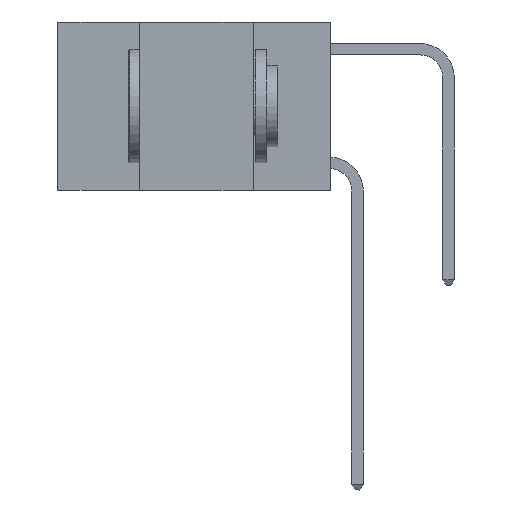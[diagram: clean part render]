
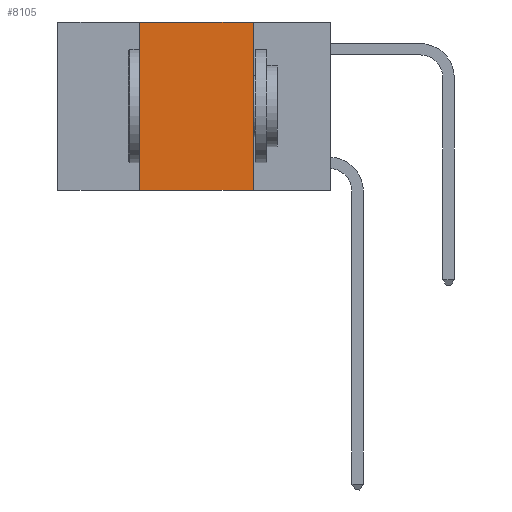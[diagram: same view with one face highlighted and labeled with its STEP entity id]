
A CAD part, left-side view. The second image highlights one B-rep face of the part: STEP entity #8105.
In plain terms, the highlighted planar face has unit normal (-1, 0, 0).
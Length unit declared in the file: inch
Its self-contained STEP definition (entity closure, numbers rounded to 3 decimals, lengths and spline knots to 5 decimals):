
#269 = AXIS2_PLACEMENT_3D ( 'NONE', #4204, #8703, #8562 ) ;
#290 = EDGE_CURVE ( 'NONE', #4850, #4384, #436, .T. ) ;
#292 = CARTESIAN_POINT ( 'NONE',  ( 0., 0.42, 0. ) ) ;
#436 = LINE ( 'NONE', #7970, #7069 ) ;
#899 = CARTESIAN_POINT ( 'NONE',  ( 0., 0.17, -0.37 ) ) ;
#1706 = FACE_OUTER_BOUND ( 'NONE', #11577, .T. ) ;
#1757 = DIRECTION ( 'NONE',  ( 0., -1., 0. ) ) ;
#2631 = VECTOR ( 'NONE', #13440, 39.37008 ) ;
#3160 = LINE ( 'NONE', #3222, #9544 ) ;
#3222 = CARTESIAN_POINT ( 'NONE',  ( 0., 0.17, 0. ) ) ;
#3410 = EDGE_CURVE ( 'NONE', #4384, #8283, #3160, .T. ) ;
#3772 = CARTESIAN_POINT ( 'NONE',  ( 0., 0.42, -0.37 ) ) ;
#3857 = ORIENTED_EDGE ( 'NONE', *, *, #9195, .T. ) ;
#4204 = CARTESIAN_POINT ( 'NONE',  ( 0., 0.6, 0. ) ) ;
#4384 = VERTEX_POINT ( 'NONE', #8143 ) ;
#4597 = CARTESIAN_POINT ( 'NONE',  ( 0., 0.6, -0.37 ) ) ;
#4850 = VERTEX_POINT ( 'NONE', #292 ) ;
#5659 = EDGE_CURVE ( 'NONE', #13352, #4850, #10112, .T. ) ;
#5739 = ORIENTED_EDGE ( 'NONE', *, *, #5659, .F. ) ;
#5869 = CARTESIAN_POINT ( 'NONE',  ( 0., 0.42, 0. ) ) ;
#6570 = PLANE ( 'NONE',  #269 ) ;
#7069 = VECTOR ( 'NONE', #1757, 39.37008 ) ;
#7970 = CARTESIAN_POINT ( 'NONE',  ( 0., 0.6, 0. ) ) ;
#8103 = DIRECTION ( 'NONE',  ( 0., 0., 1. ) ) ;
#8105 = ADVANCED_FACE ( 'NONE', ( #1706 ), #6570, .F. ) ;
#8143 = CARTESIAN_POINT ( 'NONE',  ( 0., 0.17, 0. ) ) ;
#8283 = VERTEX_POINT ( 'NONE', #899 ) ;
#8562 = DIRECTION ( 'NONE',  ( 0., 0., -1. ) ) ;
#8687 = VECTOR ( 'NONE', #8103, 39.37008 ) ;
#8703 = DIRECTION ( 'NONE',  ( 1., 0., 0. ) ) ;
#8732 = LINE ( 'NONE', #4597, #2631 ) ;
#8932 = ORIENTED_EDGE ( 'NONE', *, *, #3410, .F. ) ;
#9195 = EDGE_CURVE ( 'NONE', #13352, #8283, #8732, .T. ) ;
#9544 = VECTOR ( 'NONE', #13186, 39.37008 ) ;
#10112 = LINE ( 'NONE', #5869, #8687 ) ;
#11577 = EDGE_LOOP ( 'NONE', ( #8932, #12268, #5739, #3857 ) ) ;
#12268 = ORIENTED_EDGE ( 'NONE', *, *, #290, .F. ) ;
#13186 = DIRECTION ( 'NONE',  ( 0., 0., -1. ) ) ;
#13352 = VERTEX_POINT ( 'NONE', #3772 ) ;
#13440 = DIRECTION ( 'NONE',  ( 0., -1., 0. ) ) ;
